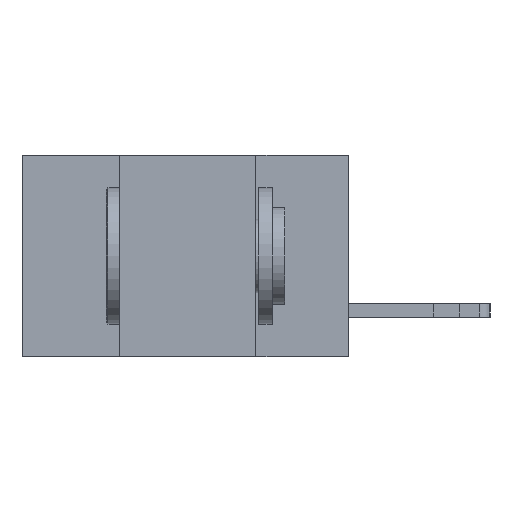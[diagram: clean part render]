
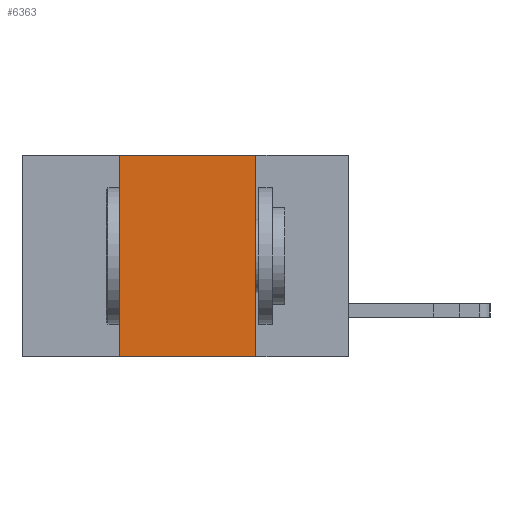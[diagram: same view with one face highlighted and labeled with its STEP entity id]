
A CAD part, left-side view. The second image highlights one B-rep face of the part: STEP entity #6363.
In plain terms, the highlighted planar face has unit normal (-1, 0, 0).
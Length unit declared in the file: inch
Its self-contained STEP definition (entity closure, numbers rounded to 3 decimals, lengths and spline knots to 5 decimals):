
#28 = AXIS2_PLACEMENT_3D ( 'NONE', #9832, #489, #1128 ) ;
#489 = DIRECTION ( 'NONE',  ( 1., 0., 0. ) ) ;
#582 = EDGE_CURVE ( 'NONE', #6943, #9868, #11704, .T. ) ;
#918 = ORIENTED_EDGE ( 'NONE', *, *, #582, .F. ) ;
#1128 = DIRECTION ( 'NONE',  ( 0., 0., -1. ) ) ;
#1688 = EDGE_LOOP ( 'NONE', ( #4891, #10849, #918, #1827 ) ) ;
#1827 = ORIENTED_EDGE ( 'NONE', *, *, #7905, .T. ) ;
#2890 = VECTOR ( 'NONE', #9035, 39.37008 ) ;
#3198 = LINE ( 'NONE', #6229, #2890 ) ;
#3329 = LINE ( 'NONE', #9932, #8131 ) ;
#3750 = VERTEX_POINT ( 'NONE', #4446 ) ;
#4446 = CARTESIAN_POINT ( 'NONE',  ( 0., 0.17, -0.37 ) ) ;
#4891 = ORIENTED_EDGE ( 'NONE', *, *, #11798, .F. ) ;
#5055 = PLANE ( 'NONE',  #28 ) ;
#5312 = DIRECTION ( 'NONE',  ( 0., -1., 0. ) ) ;
#5383 = CARTESIAN_POINT ( 'NONE',  ( 0., 0.17, 0. ) ) ;
#5384 = VERTEX_POINT ( 'NONE', #5383 ) ;
#5641 = EDGE_CURVE ( 'NONE', #9868, #5384, #7885, .T. ) ;
#6229 = CARTESIAN_POINT ( 'NONE',  ( 0., 0.17, 0. ) ) ;
#6363 = ADVANCED_FACE ( 'NONE', ( #8739 ), #5055, .F. ) ;
#6943 = VERTEX_POINT ( 'NONE', #12081 ) ;
#7203 = CARTESIAN_POINT ( 'NONE',  ( 0., 0.6, 0. ) ) ;
#7885 = LINE ( 'NONE', #7203, #9742 ) ;
#7905 = EDGE_CURVE ( 'NONE', #6943, #3750, #3329, .T. ) ;
#8131 = VECTOR ( 'NONE', #5312, 39.37008 ) ;
#8739 = FACE_OUTER_BOUND ( 'NONE', #1688, .T. ) ;
#9035 = DIRECTION ( 'NONE',  ( 0., 0., -1. ) ) ;
#9066 = DIRECTION ( 'NONE',  ( 0., -1., 0. ) ) ;
#9742 = VECTOR ( 'NONE', #9066, 39.37008 ) ;
#9832 = CARTESIAN_POINT ( 'NONE',  ( 0., 0.6, 0. ) ) ;
#9868 = VERTEX_POINT ( 'NONE', #10126 ) ;
#9932 = CARTESIAN_POINT ( 'NONE',  ( 0., 0.6, -0.37 ) ) ;
#10126 = CARTESIAN_POINT ( 'NONE',  ( 0., 0.42, 0. ) ) ;
#10849 = ORIENTED_EDGE ( 'NONE', *, *, #5641, .F. ) ;
#11139 = VECTOR ( 'NONE', #11295, 39.37008 ) ;
#11295 = DIRECTION ( 'NONE',  ( 0., 0., 1. ) ) ;
#11413 = CARTESIAN_POINT ( 'NONE',  ( 0., 0.42, 0. ) ) ;
#11704 = LINE ( 'NONE', #11413, #11139 ) ;
#11798 = EDGE_CURVE ( 'NONE', #5384, #3750, #3198, .T. ) ;
#12081 = CARTESIAN_POINT ( 'NONE',  ( 0., 0.42, -0.37 ) ) ;
